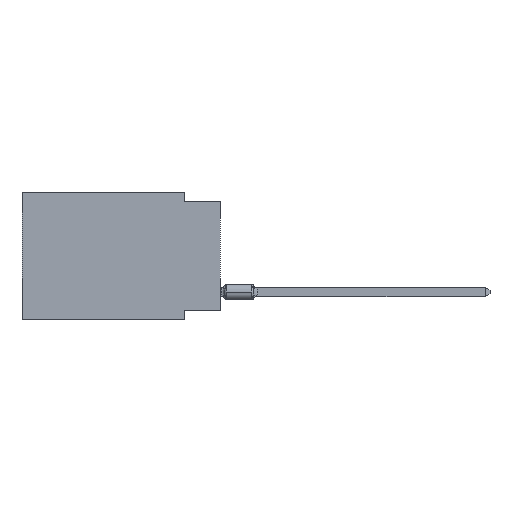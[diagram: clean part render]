
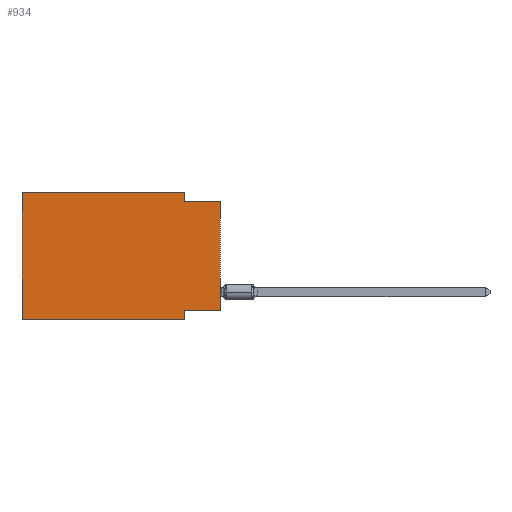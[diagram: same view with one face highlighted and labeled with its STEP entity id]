
A CAD part, left-side view. The second image highlights one B-rep face of the part: STEP entity #934.
In plain terms, the highlighted planar face has unit normal (-1, 0, 0).
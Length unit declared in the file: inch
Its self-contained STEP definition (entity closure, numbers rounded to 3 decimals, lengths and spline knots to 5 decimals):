
#158 = PLANE ( 'NONE',  #2436 ) ;
#693 = DIRECTION ( 'NONE',  ( 0., 0., -1. ) ) ;
#921 = CARTESIAN_POINT ( 'NONE',  ( 0., 0.55, 0. ) ) ;
#934 = ADVANCED_FACE ( 'NONE', ( #4423 ), #158, .F. ) ;
#1132 = CARTESIAN_POINT ( 'NONE',  ( 0., 0., -0.325 ) ) ;
#1831 = CARTESIAN_POINT ( 'NONE',  ( 0., 0., -0.025 ) ) ;
#1881 = ORIENTED_EDGE ( 'NONE', *, *, #20854, .F. ) ;
#2436 = AXIS2_PLACEMENT_3D ( 'NONE', #13093, #5030, #16328 ) ;
#2507 = EDGE_CURVE ( 'NONE', #3728, #15088, #11724, .T. ) ;
#2585 = CARTESIAN_POINT ( 'NONE',  ( 0., 0.55, 0. ) ) ;
#2899 = VECTOR ( 'NONE', #4060, 39.37008 ) ;
#3728 = VERTEX_POINT ( 'NONE', #6568 ) ;
#3778 = CARTESIAN_POINT ( 'NONE',  ( 0., 0.55, -0.35 ) ) ;
#4060 = DIRECTION ( 'NONE',  ( 0., 1., 0. ) ) ;
#4107 = EDGE_CURVE ( 'NONE', #20585, #7342, #9800, .T. ) ;
#4332 = ORIENTED_EDGE ( 'NONE', *, *, #5510, .T. ) ;
#4374 = ORIENTED_EDGE ( 'NONE', *, *, #7804, .F. ) ;
#4423 = FACE_OUTER_BOUND ( 'NONE', #14619, .T. ) ;
#5030 = DIRECTION ( 'NONE',  ( 1., 0., 0. ) ) ;
#5074 = VERTEX_POINT ( 'NONE', #12226 ) ;
#5424 = DIRECTION ( 'NONE',  ( 0., -1., 0. ) ) ;
#5510 = EDGE_CURVE ( 'NONE', #12795, #18114, #17789, .T. ) ;
#5519 = VECTOR ( 'NONE', #14057, 39.37008 ) ;
#5618 = EDGE_CURVE ( 'NONE', #20585, #15459, #15315, .T. ) ;
#5799 = DIRECTION ( 'NONE',  ( 0., 0., 1. ) ) ;
#6568 = CARTESIAN_POINT ( 'NONE',  ( 0., 0.55, 0. ) ) ;
#6601 = LINE ( 'NONE', #17481, #10927 ) ;
#6735 = VECTOR ( 'NONE', #693, 39.37008 ) ;
#6736 = CARTESIAN_POINT ( 'NONE',  ( 0., 0., -0.025 ) ) ;
#7342 = VERTEX_POINT ( 'NONE', #6736 ) ;
#7804 = EDGE_CURVE ( 'NONE', #15459, #18114, #6601, .T. ) ;
#7840 = DIRECTION ( 'NONE',  ( 0., 0., -1. ) ) ;
#8243 = CARTESIAN_POINT ( 'NONE',  ( 0., 0.55, -0.35 ) ) ;
#9050 = CARTESIAN_POINT ( 'NONE',  ( 0., 0.1, -0.325 ) ) ;
#9325 = LINE ( 'NONE', #1831, #15423 ) ;
#9384 = LINE ( 'NONE', #921, #15479 ) ;
#9671 = EDGE_CURVE ( 'NONE', #15088, #5074, #19073, .T. ) ;
#9800 = LINE ( 'NONE', #10747, #5519 ) ;
#9908 = ORIENTED_EDGE ( 'NONE', *, *, #5618, .F. ) ;
#10747 = CARTESIAN_POINT ( 'NONE',  ( 0., 0., 0. ) ) ;
#10927 = VECTOR ( 'NONE', #7840, 39.37008 ) ;
#11724 = LINE ( 'NONE', #2585, #15496 ) ;
#12226 = CARTESIAN_POINT ( 'NONE',  ( 0., 0.1, -0.025 ) ) ;
#12795 = VERTEX_POINT ( 'NONE', #8243 ) ;
#13038 = VECTOR ( 'NONE', #5424, 39.37008 ) ;
#13093 = CARTESIAN_POINT ( 'NONE',  ( 0., 0.55, 0. ) ) ;
#13292 = CARTESIAN_POINT ( 'NONE',  ( 0., 0.1, -0.35 ) ) ;
#14057 = DIRECTION ( 'NONE',  ( 0., 0., 1. ) ) ;
#14418 = ORIENTED_EDGE ( 'NONE', *, *, #2507, .F. ) ;
#14619 = EDGE_LOOP ( 'NONE', ( #20379, #1881, #16685, #14418, #20627, #4332, #4374, #9908 ) ) ;
#15088 = VERTEX_POINT ( 'NONE', #19292 ) ;
#15315 = LINE ( 'NONE', #18581, #2899 ) ;
#15423 = VECTOR ( 'NONE', #19505, 39.37008 ) ;
#15459 = VERTEX_POINT ( 'NONE', #9050 ) ;
#15479 = VECTOR ( 'NONE', #5799, 39.37008 ) ;
#15496 = VECTOR ( 'NONE', #15592, 39.37008 ) ;
#15592 = DIRECTION ( 'NONE',  ( 0., -1., 0. ) ) ;
#16328 = DIRECTION ( 'NONE',  ( 0., 0., -1. ) ) ;
#16685 = ORIENTED_EDGE ( 'NONE', *, *, #9671, .F. ) ;
#16850 = CARTESIAN_POINT ( 'NONE',  ( 0., 0.1, 0. ) ) ;
#17481 = CARTESIAN_POINT ( 'NONE',  ( 0., 0.1, -0.35 ) ) ;
#17789 = LINE ( 'NONE', #3778, #13038 ) ;
#18114 = VERTEX_POINT ( 'NONE', #13292 ) ;
#18581 = CARTESIAN_POINT ( 'NONE',  ( 0., 0., -0.325 ) ) ;
#18858 = EDGE_CURVE ( 'NONE', #12795, #3728, #9384, .T. ) ;
#19073 = LINE ( 'NONE', #16850, #6735 ) ;
#19292 = CARTESIAN_POINT ( 'NONE',  ( 0., 0.1, 0. ) ) ;
#19505 = DIRECTION ( 'NONE',  ( 0., -1., 0. ) ) ;
#20379 = ORIENTED_EDGE ( 'NONE', *, *, #4107, .T. ) ;
#20585 = VERTEX_POINT ( 'NONE', #1132 ) ;
#20627 = ORIENTED_EDGE ( 'NONE', *, *, #18858, .F. ) ;
#20854 = EDGE_CURVE ( 'NONE', #5074, #7342, #9325, .T. ) ;
